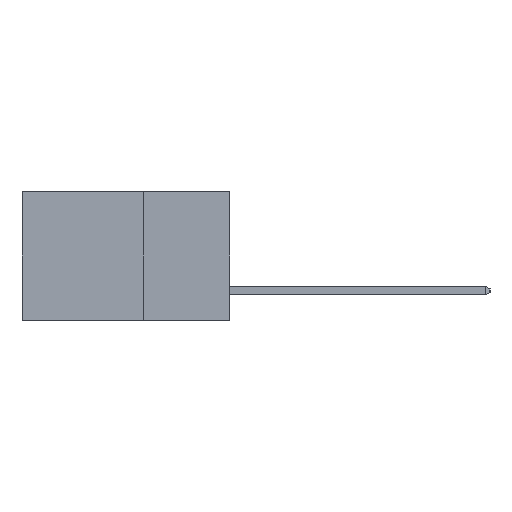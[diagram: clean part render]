
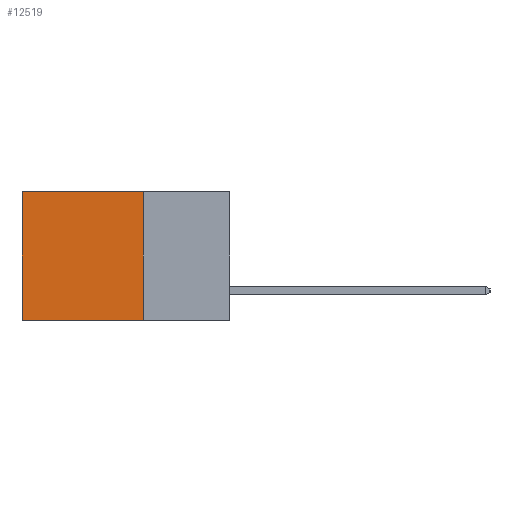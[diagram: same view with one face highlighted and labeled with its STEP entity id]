
A CAD part, left-side view. The second image highlights one B-rep face of the part: STEP entity #12519.
In plain terms, the highlighted planar face has unit normal (-1, 0, 0).
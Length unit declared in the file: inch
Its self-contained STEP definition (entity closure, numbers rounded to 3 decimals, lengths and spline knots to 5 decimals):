
#1338 = DIRECTION ( 'NONE',  ( 0., 0., -1. ) ) ;
#2095 = PLANE ( 'NONE',  #5817 ) ;
#2492 = EDGE_LOOP ( 'NONE', ( #11729, #8460, #10889, #7813 ) ) ;
#2883 = VECTOR ( 'NONE', #8167, 39.37008 ) ;
#3065 = DIRECTION ( 'NONE',  ( 0., 1., 0. ) ) ;
#3656 = FACE_OUTER_BOUND ( 'NONE', #2492, .T. ) ;
#3703 = VECTOR ( 'NONE', #3065, 39.37008 ) ;
#3884 = CARTESIAN_POINT ( 'NONE',  ( 0.298, 0.25, 0. ) ) ;
#4147 = DIRECTION ( 'NONE',  ( 1., 0., 0. ) ) ;
#4889 = VECTOR ( 'NONE', #19788, 39.37008 ) ;
#5817 = AXIS2_PLACEMENT_3D ( 'NONE', #10043, #4147, #18129 ) ;
#5822 = VERTEX_POINT ( 'NONE', #22615 ) ;
#6149 = CARTESIAN_POINT ( 'NONE',  ( 0.298, 0.25, 0. ) ) ;
#6919 = EDGE_CURVE ( 'NONE', #19535, #12537, #18868, .T. ) ;
#7813 = ORIENTED_EDGE ( 'NONE', *, *, #17560, .T. ) ;
#8167 = DIRECTION ( 'NONE',  ( 0., 0., -1. ) ) ;
#8460 = ORIENTED_EDGE ( 'NONE', *, *, #15963, .F. ) ;
#9890 = EDGE_CURVE ( 'NONE', #5822, #12977, #24808, .T. ) ;
#10043 = CARTESIAN_POINT ( 'NONE',  ( 0.298, 0.25, 0. ) ) ;
#10889 = ORIENTED_EDGE ( 'NONE', *, *, #6919, .F. ) ;
#11604 = CARTESIAN_POINT ( 'NONE',  ( 0.298, 0.6, -0.37 ) ) ;
#11729 = ORIENTED_EDGE ( 'NONE', *, *, #9890, .T. ) ;
#12519 = ADVANCED_FACE ( 'NONE', ( #3656 ), #2095, .F. ) ;
#12537 = VERTEX_POINT ( 'NONE', #18216 ) ;
#12977 = VERTEX_POINT ( 'NONE', #11604 ) ;
#15115 = CARTESIAN_POINT ( 'NONE',  ( 0.298, 0.25, -0.37 ) ) ;
#15554 = LINE ( 'NONE', #3884, #4889 ) ;
#15963 = EDGE_CURVE ( 'NONE', #12537, #12977, #19048, .T. ) ;
#17560 = EDGE_CURVE ( 'NONE', #19535, #5822, #15554, .T. ) ;
#18129 = DIRECTION ( 'NONE',  ( 0., 0., -1. ) ) ;
#18216 = CARTESIAN_POINT ( 'NONE',  ( 0.298, 0.25, -0.37 ) ) ;
#18868 = LINE ( 'NONE', #6149, #2883 ) ;
#19048 = LINE ( 'NONE', #15115, #3703 ) ;
#19399 = CARTESIAN_POINT ( 'NONE',  ( 0.298, 0.25, 0. ) ) ;
#19535 = VERTEX_POINT ( 'NONE', #19399 ) ;
#19759 = VECTOR ( 'NONE', #1338, 39.37008 ) ;
#19788 = DIRECTION ( 'NONE',  ( 0., 1., 0. ) ) ;
#21267 = CARTESIAN_POINT ( 'NONE',  ( 0.298, 0.6, 0. ) ) ;
#22615 = CARTESIAN_POINT ( 'NONE',  ( 0.298, 0.6, 0. ) ) ;
#24808 = LINE ( 'NONE', #21267, #19759 ) ;
